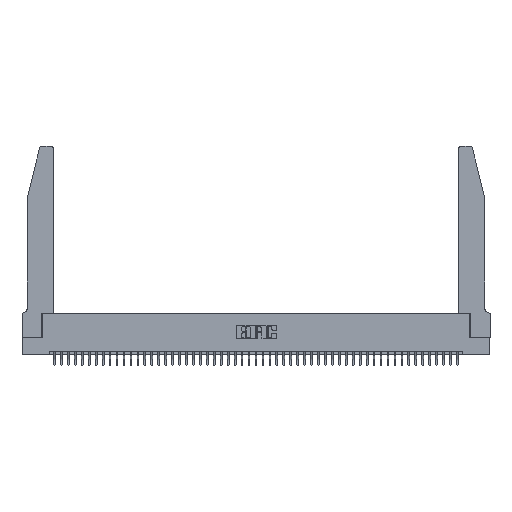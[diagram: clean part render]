
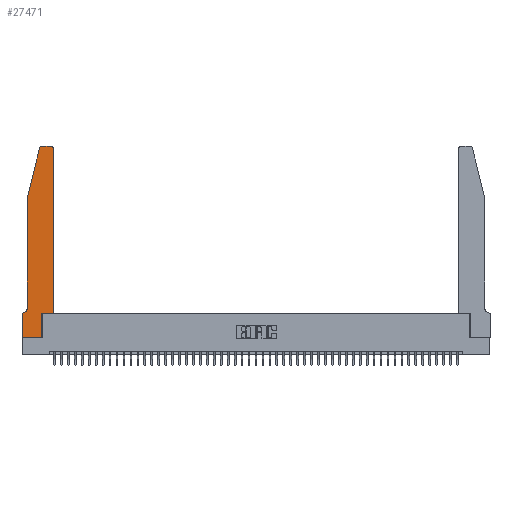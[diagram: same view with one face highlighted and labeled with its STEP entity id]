
A CAD part, top view. The second image highlights one B-rep face of the part: STEP entity #27471.
In plain terms, the highlighted planar face has unit normal (0, 0, 1).
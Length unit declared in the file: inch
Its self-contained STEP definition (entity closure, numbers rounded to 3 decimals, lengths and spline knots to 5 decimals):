
#189 = ORIENTED_EDGE ( 'NONE', *, *, #34501, .T. ) ;
#484 = CARTESIAN_POINT ( 'NONE',  ( 0.0755, 2., 0.37 ) ) ;
#1532 = LINE ( 'NONE', #30379, #35418 ) ;
#2660 = CARTESIAN_POINT ( 'NONE',  ( 0.4505, 2.72, 0.37 ) ) ;
#3851 = DIRECTION ( 'NONE',  ( 1., 0., 0. ) ) ;
#4109 = CARTESIAN_POINT ( 'NONE',  ( 0.2865, 0.35, 0.37 ) ) ;
#4220 = ORIENTED_EDGE ( 'NONE', *, *, #36020, .T. ) ;
#5357 = DIRECTION ( 'NONE',  ( 0., 0., 1. ) ) ;
#7448 = VERTEX_POINT ( 'NONE', #37296 ) ;
#7834 = VERTEX_POINT ( 'NONE', #36108 ) ;
#8350 = PLANE ( 'NONE',  #25433 ) ;
#8356 = EDGE_CURVE ( 'NONE', #46466, #48418, #20651, .T. ) ;
#8550 = DIRECTION ( 'NONE',  ( 1., 0., 0. ) ) ;
#8633 = LINE ( 'NONE', #36439, #48609 ) ;
#9166 = ORIENTED_EDGE ( 'NONE', *, *, #17579, .T. ) ;
#9883 = VECTOR ( 'NONE', #14352, 39.37008 ) ;
#10685 = VERTEX_POINT ( 'NONE', #2660 ) ;
#11184 = EDGE_CURVE ( 'NONE', #7834, #10685, #8633, .T. ) ;
#11826 = CARTESIAN_POINT ( 'NONE',  ( 0., 0.35, 0.37 ) ) ;
#12072 = DIRECTION ( 'NONE',  ( 0., -1., 0. ) ) ;
#12096 = CIRCLE ( 'NONE', #13885, 0.03 ) ;
#12787 = CARTESIAN_POINT ( 'NONE',  ( 0.0755, 0.42, 0.37 ) ) ;
#13875 = EDGE_LOOP ( 'NONE', ( #25100, #27597, #22929, #4220, #28723, #189, #37692, #40102, #29180, #36156, #15390, #9166 ) ) ;
#13885 = AXIS2_PLACEMENT_3D ( 'NONE', #28053, #5357, #31836 ) ;
#13935 = DIRECTION ( 'NONE',  ( 0., 1., 0. ) ) ;
#14115 = CIRCLE ( 'NONE', #16253, 0.07 ) ;
#14352 = DIRECTION ( 'NONE',  ( -1., 0., 0. ) ) ;
#14524 = FACE_OUTER_BOUND ( 'NONE', #13875, .T. ) ;
#15390 = ORIENTED_EDGE ( 'NONE', *, *, #11184, .T. ) ;
#16007 = DIRECTION ( 'NONE',  ( 1., 0., 0. ) ) ;
#16253 = AXIS2_PLACEMENT_3D ( 'NONE', #19911, #46144, #23683 ) ;
#17325 = VERTEX_POINT ( 'NONE', #19212 ) ;
#17579 = EDGE_CURVE ( 'NONE', #10685, #41832, #12096, .T. ) ;
#18312 = LINE ( 'NONE', #44509, #47031 ) ;
#19212 = CARTESIAN_POINT ( 'NONE',  ( 0.0055, 0.35, 0.37 ) ) ;
#19911 = CARTESIAN_POINT ( 'NONE',  ( 0.0055, 0.42, 0.37 ) ) ;
#20080 = DIRECTION ( 'NONE',  ( -1., 0., 0. ) ) ;
#20423 = CARTESIAN_POINT ( 'NONE',  ( 0.284, 2.72, 0.37 ) ) ;
#20651 = CIRCLE ( 'NONE', #33450, 0.03 ) ;
#21258 = CARTESIAN_POINT ( 'NONE',  ( 0.0755, 2., 0.37 ) ) ;
#22880 = VECTOR ( 'NONE', #20080, 39.37008 ) ;
#22905 = VECTOR ( 'NONE', #28054, 39.37008 ) ;
#22929 = ORIENTED_EDGE ( 'NONE', *, *, #47161, .T. ) ;
#23683 = DIRECTION ( 'NONE',  ( -1., 0., 0. ) ) ;
#23827 = CARTESIAN_POINT ( 'NONE',  ( 0.4205, 2.75, 0.37 ) ) ;
#24209 = DIRECTION ( 'NONE',  ( 1., 0., 0. ) ) ;
#24263 = CARTESIAN_POINT ( 'NONE',  ( 0., 0., 0.37 ) ) ;
#25100 = ORIENTED_EDGE ( 'NONE', *, *, #33442, .T. ) ;
#25433 = AXIS2_PLACEMENT_3D ( 'NONE', #45844, #38524, #16007 ) ;
#25517 = CARTESIAN_POINT ( 'NONE',  ( 0.0755, 0.35, 0.37 ) ) ;
#25794 = DIRECTION ( 'NONE',  ( -0.239, -0.971, 0. ) ) ;
#27442 = CARTESIAN_POINT ( 'NONE',  ( 0.2865, 0., 0.37 ) ) ;
#27471 = ADVANCED_FACE ( 'NONE', ( #14524 ), #8350, .T. ) ;
#27597 = ORIENTED_EDGE ( 'NONE', *, *, #8356, .T. ) ;
#27641 = CARTESIAN_POINT ( 'NONE',  ( 0.2605, 2.75, 0.37 ) ) ;
#28053 = CARTESIAN_POINT ( 'NONE',  ( 0.4205, 2.72, 0.37 ) ) ;
#28054 = DIRECTION ( 'NONE',  ( 0., -1., 0. ) ) ;
#28258 = VECTOR ( 'NONE', #36728, 39.37008 ) ;
#28723 = ORIENTED_EDGE ( 'NONE', *, *, #48656, .T. ) ;
#28998 = CARTESIAN_POINT ( 'NONE',  ( 0.284, 2.75, 0.37 ) ) ;
#29180 = ORIENTED_EDGE ( 'NONE', *, *, #48311, .T. ) ;
#29758 = VERTEX_POINT ( 'NONE', #21258 ) ;
#29812 = CARTESIAN_POINT ( 'NONE',  ( 0.25487, 2.72718, 0.37 ) ) ;
#30353 = VECTOR ( 'NONE', #12072, 39.37008 ) ;
#30379 = CARTESIAN_POINT ( 'NONE',  ( 0., 0., 0.37 ) ) ;
#31836 = DIRECTION ( 'NONE',  ( 1., 0., 0. ) ) ;
#32916 = LINE ( 'NONE', #24263, #22905 ) ;
#33442 = EDGE_CURVE ( 'NONE', #41832, #46466, #35246, .T. ) ;
#33450 = AXIS2_PLACEMENT_3D ( 'NONE', #20423, #46656, #24209 ) ;
#34501 = EDGE_CURVE ( 'NONE', #17325, #37779, #38759, .T. ) ;
#34924 = CARTESIAN_POINT ( 'NONE',  ( 0.4505, 0.35, 0.37 ) ) ;
#35246 = LINE ( 'NONE', #27641, #22880 ) ;
#35418 = VECTOR ( 'NONE', #3851, 39.37008 ) ;
#36020 = EDGE_CURVE ( 'NONE', #29758, #40529, #40374, .T. ) ;
#36108 = CARTESIAN_POINT ( 'NONE',  ( 0.4505, 0.35, 0.37 ) ) ;
#36131 = LINE ( 'NONE', #34924, #47228 ) ;
#36156 = ORIENTED_EDGE ( 'NONE', *, *, #41132, .T. ) ;
#36439 = CARTESIAN_POINT ( 'NONE',  ( 0.4505, 0.35, 0.37 ) ) ;
#36567 = CARTESIAN_POINT ( 'NONE',  ( 0.2865, 0.35, 0.37 ) ) ;
#36728 = DIRECTION ( 'NONE',  ( 0., 1., 0. ) ) ;
#37296 = CARTESIAN_POINT ( 'NONE',  ( 0., 0., 0.37 ) ) ;
#37692 = ORIENTED_EDGE ( 'NONE', *, *, #38038, .T. ) ;
#37779 = VERTEX_POINT ( 'NONE', #11826 ) ;
#38038 = EDGE_CURVE ( 'NONE', #37779, #7448, #32916, .T. ) ;
#38282 = LINE ( 'NONE', #36567, #28258 ) ;
#38524 = DIRECTION ( 'NONE',  ( 0., 0., 1. ) ) ;
#38759 = LINE ( 'NONE', #25517, #9883 ) ;
#40102 = ORIENTED_EDGE ( 'NONE', *, *, #42334, .T. ) ;
#40374 = LINE ( 'NONE', #484, #30353 ) ;
#40529 = VERTEX_POINT ( 'NONE', #12787 ) ;
#41132 = EDGE_CURVE ( 'NONE', #48559, #7834, #36131, .T. ) ;
#41832 = VERTEX_POINT ( 'NONE', #23827 ) ;
#42334 = EDGE_CURVE ( 'NONE', #7448, #45584, #1532, .T. ) ;
#44509 = CARTESIAN_POINT ( 'NONE',  ( 0.0755, 2., 0.37 ) ) ;
#45584 = VERTEX_POINT ( 'NONE', #27442 ) ;
#45844 = CARTESIAN_POINT ( 'NONE',  ( 0., 0.35, 0.37 ) ) ;
#46144 = DIRECTION ( 'NONE',  ( 0., 0., -1. ) ) ;
#46466 = VERTEX_POINT ( 'NONE', #28998 ) ;
#46656 = DIRECTION ( 'NONE',  ( 0., 0., 1. ) ) ;
#47031 = VECTOR ( 'NONE', #25794, 39.37008 ) ;
#47161 = EDGE_CURVE ( 'NONE', #48418, #29758, #18312, .T. ) ;
#47228 = VECTOR ( 'NONE', #8550, 39.37008 ) ;
#48311 = EDGE_CURVE ( 'NONE', #45584, #48559, #38282, .T. ) ;
#48418 = VERTEX_POINT ( 'NONE', #29812 ) ;
#48559 = VERTEX_POINT ( 'NONE', #4109 ) ;
#48609 = VECTOR ( 'NONE', #13935, 39.37008 ) ;
#48656 = EDGE_CURVE ( 'NONE', #40529, #17325, #14115, .T. ) ;
